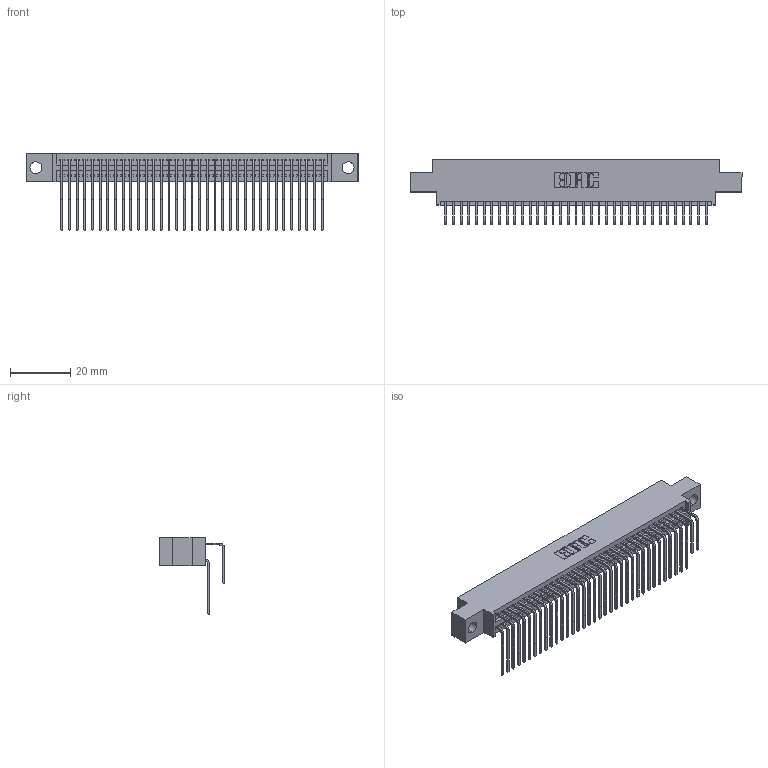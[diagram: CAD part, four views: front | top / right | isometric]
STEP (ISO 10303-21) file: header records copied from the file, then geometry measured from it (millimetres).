
FILE_DESCRIPTION (( 'STEP AP203' ), '1' );
FILE_NAME ('395-070-558-804.STEP', '2021-06-17T04:41:24', ( '' ), ( '' ), 'SwSTEP 2.0', 'SolidWorks 2020', '' );
FILE_SCHEMA (( 'CONFIG_CONTROL_DESIGN' ));
Length unit declared in the file: inch
Products named in the file (4): 345-292-001_558 559 Tail - 1; 345-292-001_558 Tail - 2; 395-070-558-804; 345 Part_0.170 Offset - 0.156 Dia-TI
Assembly tree (71 placements, depth 2):
  395-070-558-804
    345 Part_0.170 Offset - 0.156 Dia-TI
    345-292-001_558 559 Tail - 1  x35
    345-292-001_558 Tail - 2  x35
Bounding box: 110.11 x 21.83 x 25.53 mm (x, y, z)
Volume: 10815.6 mm3; surface area: 17745.6 mm2
Topology: 71 solids, 71 shells, 3784 faces, 11239 edges, 7398 vertices
Faces by surface type: plane 2548, cylinder 1236
Entity records: 30607 total; most frequent: CARTESIAN_POINT 5189, ORIENTED_EDGE 5070, DIRECTION 4555, EDGE_CURVE 2535, VECTOR 2223, LINE 2223, VERTEX_POINT 1686, AXIS2_PLACEMENT_3D 1166
